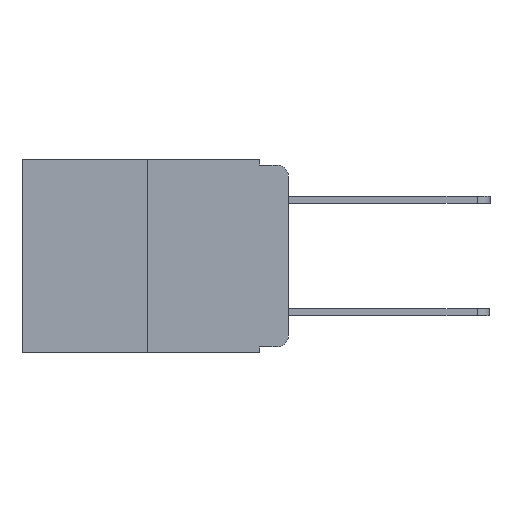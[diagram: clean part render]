
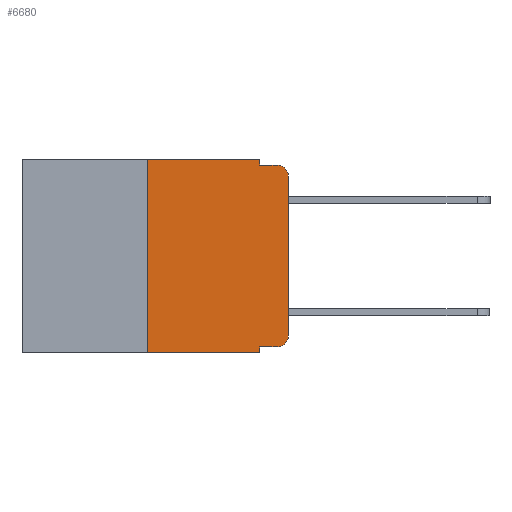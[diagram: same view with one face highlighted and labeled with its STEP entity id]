
A CAD part, left-side view. The second image highlights one B-rep face of the part: STEP entity #6680.
In plain terms, the highlighted planar face has unit normal (-1, 0, 0).
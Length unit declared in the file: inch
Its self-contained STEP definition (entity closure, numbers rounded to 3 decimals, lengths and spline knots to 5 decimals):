
#5 = LINE ( 'NONE', #9927, #10445 ) ;
#44 = ORIENTED_EDGE ( 'NONE', *, *, #3678, .F. ) ;
#432 = DIRECTION ( 'NONE',  ( 0., 0., 1. ) ) ;
#594 = ORIENTED_EDGE ( 'NONE', *, *, #6398, .T. ) ;
#797 = ORIENTED_EDGE ( 'NONE', *, *, #5488, .T. ) ;
#890 = DIRECTION ( 'NONE',  ( 0., 0., -1. ) ) ;
#970 = CARTESIAN_POINT ( 'NONE',  ( 0., 0.25, -0.343 ) ) ;
#1598 = VECTOR ( 'NONE', #1902, 39.37008 ) ;
#1694 = EDGE_CURVE ( 'NONE', #10956, #8664, #5384, .T. ) ;
#1887 = ORIENTED_EDGE ( 'NONE', *, *, #8586, .F. ) ;
#1902 = DIRECTION ( 'NONE',  ( 0., 0., 1. ) ) ;
#2011 = CARTESIAN_POINT ( 'NONE',  ( 0., 0.02, -0.333 ) ) ;
#2648 = ORIENTED_EDGE ( 'NONE', *, *, #1694, .F. ) ;
#2673 = CARTESIAN_POINT ( 'NONE',  ( 0., 0.051, -0.01 ) ) ;
#2692 = EDGE_CURVE ( 'NONE', #13768, #10319, #3858, .T. ) ;
#3007 = VECTOR ( 'NONE', #10992, 39.37008 ) ;
#3086 = AXIS2_PLACEMENT_3D ( 'NONE', #13192, #5729, #14350 ) ;
#3299 = CARTESIAN_POINT ( 'NONE',  ( 0., 0.02, -0.313 ) ) ;
#3393 = CARTESIAN_POINT ( 'NONE',  ( 0., 0.25, 0. ) ) ;
#3409 = VECTOR ( 'NONE', #890, 39.37008 ) ;
#3533 = FACE_OUTER_BOUND ( 'NONE', #7344, .T. ) ;
#3582 = VERTEX_POINT ( 'NONE', #9407 ) ;
#3678 = EDGE_CURVE ( 'NONE', #10319, #9696, #4286, .T. ) ;
#3858 = LINE ( 'NONE', #15065, #3409 ) ;
#4263 = ORIENTED_EDGE ( 'NONE', *, *, #16406, .F. ) ;
#4286 = LINE ( 'NONE', #12068, #10710 ) ;
#4335 = CARTESIAN_POINT ( 'NONE',  ( 0., 0.051, -0.333 ) ) ;
#4385 = PLANE ( 'NONE',  #6540 ) ;
#4605 = VERTEX_POINT ( 'NONE', #11067 ) ;
#4689 = DIRECTION ( 'NONE',  ( 0., 0., -1. ) ) ;
#5384 = LINE ( 'NONE', #3393, #1598 ) ;
#5488 = EDGE_CURVE ( 'NONE', #4605, #9696, #12192, .T. ) ;
#5526 = VECTOR ( 'NONE', #7229, 39.37008 ) ;
#5598 = CARTESIAN_POINT ( 'NONE',  ( 0., 0.02, -0.01 ) ) ;
#5729 = DIRECTION ( 'NONE',  ( -1., 0., 0. ) ) ;
#5753 = CARTESIAN_POINT ( 'NONE',  ( 0., 0.051, -0.333 ) ) ;
#6048 = ORIENTED_EDGE ( 'NONE', *, *, #15843, .T. ) ;
#6398 = EDGE_CURVE ( 'NONE', #11939, #4605, #5, .T. ) ;
#6540 = AXIS2_PLACEMENT_3D ( 'NONE', #12008, #13529, #9598 ) ;
#6620 = ORIENTED_EDGE ( 'NONE', *, *, #15640, .T. ) ;
#6680 = ADVANCED_FACE ( 'NONE', ( #3533 ), #4385, .F. ) ;
#6798 = ORIENTED_EDGE ( 'NONE', *, *, #14879, .T. ) ;
#7229 = DIRECTION ( 'NONE',  ( 0., -1., 0. ) ) ;
#7344 = EDGE_LOOP ( 'NONE', ( #594, #797, #44, #15997, #1887, #2648, #6048, #4263, #6620, #6798 ) ) ;
#8191 = CARTESIAN_POINT ( 'NONE',  ( 0., 0.051, 0. ) ) ;
#8267 = CIRCLE ( 'NONE', #10771, 0.02 ) ;
#8451 = LINE ( 'NONE', #4335, #14444 ) ;
#8509 = CARTESIAN_POINT ( 'NONE',  ( 0., 0.473, 0. ) ) ;
#8586 = EDGE_CURVE ( 'NONE', #8664, #13768, #8992, .T. ) ;
#8610 = CARTESIAN_POINT ( 'NONE',  ( 0., 0.25, 0. ) ) ;
#8664 = VERTEX_POINT ( 'NONE', #8610 ) ;
#8992 = LINE ( 'NONE', #8509, #5526 ) ;
#9218 = LINE ( 'NONE', #11894, #12070 ) ;
#9407 = CARTESIAN_POINT ( 'NONE',  ( 0., 0.051, -0.343 ) ) ;
#9598 = DIRECTION ( 'NONE',  ( 0., 0., -1. ) ) ;
#9696 = VERTEX_POINT ( 'NONE', #5598 ) ;
#9927 = CARTESIAN_POINT ( 'NONE',  ( 0., 0., 0. ) ) ;
#10319 = VERTEX_POINT ( 'NONE', #2673 ) ;
#10445 = VECTOR ( 'NONE', #432, 39.37008 ) ;
#10636 = VERTEX_POINT ( 'NONE', #2011 ) ;
#10710 = VECTOR ( 'NONE', #10880, 39.37008 ) ;
#10771 = AXIS2_PLACEMENT_3D ( 'NONE', #3299, #12269, #4689 ) ;
#10880 = DIRECTION ( 'NONE',  ( 0., -1., 0. ) ) ;
#10956 = VERTEX_POINT ( 'NONE', #970 ) ;
#10992 = DIRECTION ( 'NONE',  ( 0., -1., 0. ) ) ;
#11067 = CARTESIAN_POINT ( 'NONE',  ( 0., 0., -0.03 ) ) ;
#11894 = CARTESIAN_POINT ( 'NONE',  ( 0., 0.051, 0. ) ) ;
#11939 = VERTEX_POINT ( 'NONE', #13126 ) ;
#12008 = CARTESIAN_POINT ( 'NONE',  ( 0., 0.473, 0. ) ) ;
#12068 = CARTESIAN_POINT ( 'NONE',  ( 0., 0.051, -0.01 ) ) ;
#12070 = VECTOR ( 'NONE', #13077, 39.37008 ) ;
#12192 = CIRCLE ( 'NONE', #3086, 0.02 ) ;
#12269 = DIRECTION ( 'NONE',  ( -1., 0., 0. ) ) ;
#12744 = VERTEX_POINT ( 'NONE', #5753 ) ;
#13077 = DIRECTION ( 'NONE',  ( 0., 0., -1. ) ) ;
#13126 = CARTESIAN_POINT ( 'NONE',  ( 0., 0., -0.313 ) ) ;
#13192 = CARTESIAN_POINT ( 'NONE',  ( 0., 0.02, -0.03 ) ) ;
#13193 = LINE ( 'NONE', #15718, #3007 ) ;
#13529 = DIRECTION ( 'NONE',  ( 1., 0., 0. ) ) ;
#13768 = VERTEX_POINT ( 'NONE', #8191 ) ;
#14308 = DIRECTION ( 'NONE',  ( 0., -1., 0. ) ) ;
#14350 = DIRECTION ( 'NONE',  ( 0., 0., -1. ) ) ;
#14444 = VECTOR ( 'NONE', #14308, 39.37008 ) ;
#14879 = EDGE_CURVE ( 'NONE', #10636, #11939, #8267, .T. ) ;
#15065 = CARTESIAN_POINT ( 'NONE',  ( 0., 0.051, 0. ) ) ;
#15640 = EDGE_CURVE ( 'NONE', #12744, #10636, #8451, .T. ) ;
#15718 = CARTESIAN_POINT ( 'NONE',  ( 0., 0.473, -0.343 ) ) ;
#15843 = EDGE_CURVE ( 'NONE', #10956, #3582, #13193, .T. ) ;
#15997 = ORIENTED_EDGE ( 'NONE', *, *, #2692, .F. ) ;
#16406 = EDGE_CURVE ( 'NONE', #12744, #3582, #9218, .T. ) ;
